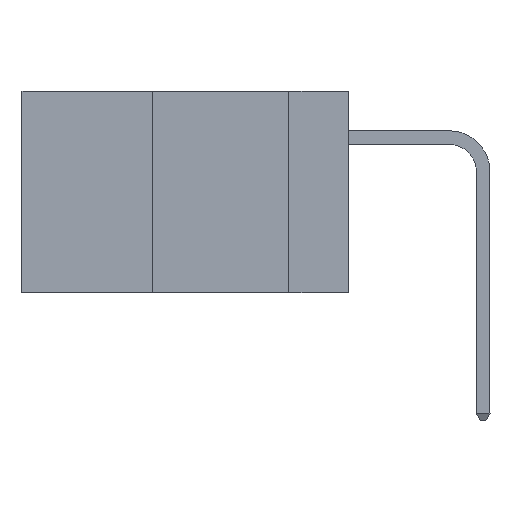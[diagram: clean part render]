
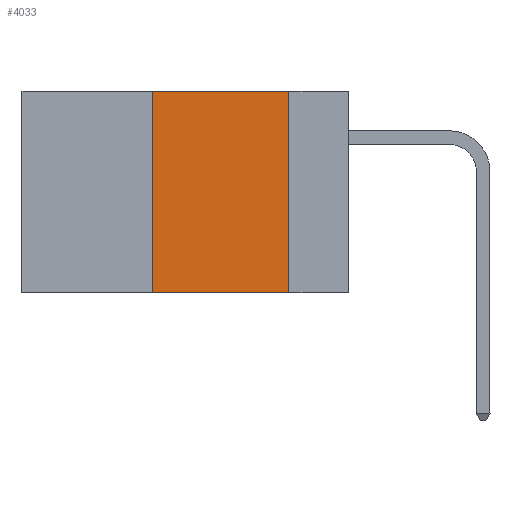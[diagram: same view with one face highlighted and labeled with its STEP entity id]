
A CAD part, left-side view. The second image highlights one B-rep face of the part: STEP entity #4033.
In plain terms, the highlighted planar face has unit normal (-1, 0, 0).
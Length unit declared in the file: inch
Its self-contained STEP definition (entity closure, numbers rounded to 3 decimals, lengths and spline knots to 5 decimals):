
#45 = CARTESIAN_POINT ( 'NONE',  ( 0., 0.11, 0. ) ) ;
#790 = EDGE_CURVE ( 'NONE', #12275, #1332, #9162, .T. ) ;
#910 = CARTESIAN_POINT ( 'NONE',  ( 0., 0.36, -0.37 ) ) ;
#1332 = VERTEX_POINT ( 'NONE', #8465 ) ;
#1423 = VECTOR ( 'NONE', #4133, 39.37008 ) ;
#1449 = VECTOR ( 'NONE', #14664, 39.37008 ) ;
#2013 = VECTOR ( 'NONE', #11442, 39.37008 ) ;
#2034 = AXIS2_PLACEMENT_3D ( 'NONE', #8333, #5826, #3380 ) ;
#2799 = LINE ( 'NONE', #8122, #1423 ) ;
#3380 = DIRECTION ( 'NONE',  ( 0., 0., -1. ) ) ;
#3415 = EDGE_CURVE ( 'NONE', #13641, #10883, #2799, .T. ) ;
#4033 = ADVANCED_FACE ( 'NONE', ( #5739 ), #4710, .F. ) ;
#4133 = DIRECTION ( 'NONE',  ( 0., 0., -1. ) ) ;
#4710 = PLANE ( 'NONE',  #2034 ) ;
#5739 = FACE_OUTER_BOUND ( 'NONE', #8213, .T. ) ;
#5826 = DIRECTION ( 'NONE',  ( 1., 0., 0. ) ) ;
#6084 = ORIENTED_EDGE ( 'NONE', *, *, #3415, .F. ) ;
#7696 = ORIENTED_EDGE ( 'NONE', *, *, #790, .F. ) ;
#7732 = LINE ( 'NONE', #12624, #14846 ) ;
#8122 = CARTESIAN_POINT ( 'NONE',  ( 0., 0.11, 0. ) ) ;
#8213 = EDGE_LOOP ( 'NONE', ( #6084, #9794, #7696, #12135 ) ) ;
#8333 = CARTESIAN_POINT ( 'NONE',  ( 0., 0.6, 0. ) ) ;
#8465 = CARTESIAN_POINT ( 'NONE',  ( 0., 0.36, 0. ) ) ;
#8797 = EDGE_CURVE ( 'NONE', #1332, #13641, #7732, .T. ) ;
#8927 = CARTESIAN_POINT ( 'NONE',  ( 0., 0.36, 0. ) ) ;
#9162 = LINE ( 'NONE', #8927, #2013 ) ;
#9794 = ORIENTED_EDGE ( 'NONE', *, *, #8797, .F. ) ;
#10883 = VERTEX_POINT ( 'NONE', #12191 ) ;
#11275 = DIRECTION ( 'NONE',  ( 0., -1., 0. ) ) ;
#11442 = DIRECTION ( 'NONE',  ( 0., 0., 1. ) ) ;
#11479 = CARTESIAN_POINT ( 'NONE',  ( 0., 0.6, -0.37 ) ) ;
#12135 = ORIENTED_EDGE ( 'NONE', *, *, #14653, .T. ) ;
#12191 = CARTESIAN_POINT ( 'NONE',  ( 0., 0.11, -0.37 ) ) ;
#12275 = VERTEX_POINT ( 'NONE', #910 ) ;
#12624 = CARTESIAN_POINT ( 'NONE',  ( 0., 0.6, 0. ) ) ;
#13641 = VERTEX_POINT ( 'NONE', #45 ) ;
#14653 = EDGE_CURVE ( 'NONE', #12275, #10883, #15111, .T. ) ;
#14664 = DIRECTION ( 'NONE',  ( 0., -1., 0. ) ) ;
#14846 = VECTOR ( 'NONE', #11275, 39.37008 ) ;
#15111 = LINE ( 'NONE', #11479, #1449 ) ;
